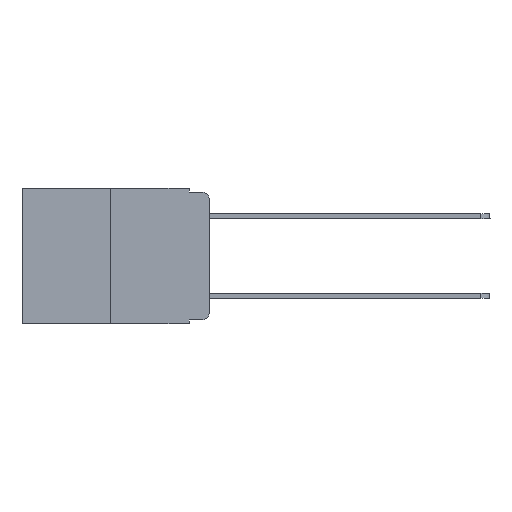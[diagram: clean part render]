
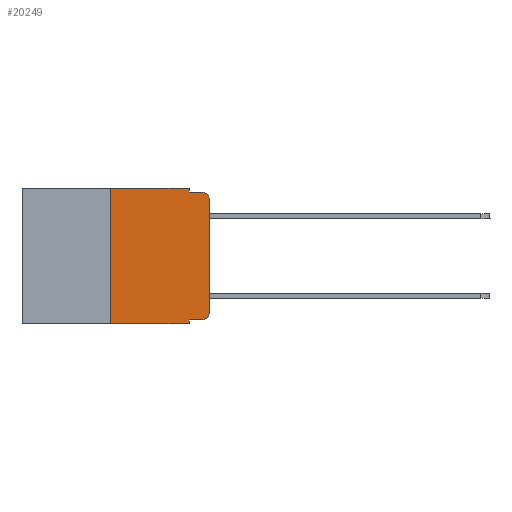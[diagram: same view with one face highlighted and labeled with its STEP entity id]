
A CAD part, left-side view. The second image highlights one B-rep face of the part: STEP entity #20249.
In plain terms, the highlighted planar face has unit normal (-1, 0, 0).
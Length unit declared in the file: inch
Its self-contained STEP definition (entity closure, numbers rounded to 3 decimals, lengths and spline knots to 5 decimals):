
#166 = ORIENTED_EDGE ( 'NONE', *, *, #11618, .F. ) ;
#709 = DIRECTION ( 'NONE',  ( 0., 0., -1. ) ) ;
#1634 = LINE ( 'NONE', #14642, #17639 ) ;
#1805 = DIRECTION ( 'NONE',  ( 0., 0., -1. ) ) ;
#2000 = CARTESIAN_POINT ( 'NONE',  ( 0., 0.473, 0. ) ) ;
#2023 = CARTESIAN_POINT ( 'NONE',  ( 0., 0.25, -0.343 ) ) ;
#2634 = DIRECTION ( 'NONE',  ( 0., -1., 0. ) ) ;
#2827 = CARTESIAN_POINT ( 'NONE',  ( 0., 0.25, 0. ) ) ;
#2883 = CARTESIAN_POINT ( 'NONE',  ( 0., 0.051, -0.343 ) ) ;
#2900 = CARTESIAN_POINT ( 'NONE',  ( 0., 0.051, -0.333 ) ) ;
#2901 = CARTESIAN_POINT ( 'NONE',  ( 0., 0.02, -0.333 ) ) ;
#3728 = CARTESIAN_POINT ( 'NONE',  ( 0., 0., -0.313 ) ) ;
#3731 = CIRCLE ( 'NONE', #4537, 0.02 ) ;
#3803 = ORIENTED_EDGE ( 'NONE', *, *, #8264, .F. ) ;
#3992 = VERTEX_POINT ( 'NONE', #2901 ) ;
#4128 = DIRECTION ( 'NONE',  ( -1., 0., 0. ) ) ;
#4416 = CARTESIAN_POINT ( 'NONE',  ( 0., 0.02, -0.313 ) ) ;
#4537 = AXIS2_PLACEMENT_3D ( 'NONE', #4416, #4580, #709 ) ;
#4580 = DIRECTION ( 'NONE',  ( -1., 0., 0. ) ) ;
#5114 = ORIENTED_EDGE ( 'NONE', *, *, #7189, .F. ) ;
#5396 = CARTESIAN_POINT ( 'NONE',  ( 0., 0.051, 0. ) ) ;
#5614 = EDGE_CURVE ( 'NONE', #18239, #15077, #23805, .T. ) ;
#6488 = DIRECTION ( 'NONE',  ( 0., -1., 0. ) ) ;
#6536 = ORIENTED_EDGE ( 'NONE', *, *, #17992, .F. ) ;
#6770 = DIRECTION ( 'NONE',  ( 0., 0., -1. ) ) ;
#6808 = ORIENTED_EDGE ( 'NONE', *, *, #16157, .F. ) ;
#7189 = EDGE_CURVE ( 'NONE', #14477, #15077, #16573, .T. ) ;
#8081 = CARTESIAN_POINT ( 'NONE',  ( 0., 0.25, 0. ) ) ;
#8264 = EDGE_CURVE ( 'NONE', #18609, #8531, #9358, .T. ) ;
#8531 = VERTEX_POINT ( 'NONE', #2883 ) ;
#8640 = VERTEX_POINT ( 'NONE', #3728 ) ;
#8918 = LINE ( 'NONE', #8081, #15441 ) ;
#8954 = DIRECTION ( 'NONE',  ( 0., 0., 1. ) ) ;
#9109 = CARTESIAN_POINT ( 'NONE',  ( 0., 0., 0. ) ) ;
#9358 = LINE ( 'NONE', #5396, #10633 ) ;
#10253 = DIRECTION ( 'NONE',  ( 0., 0., 1. ) ) ;
#10358 = CARTESIAN_POINT ( 'NONE',  ( 0., 0.051, -0.333 ) ) ;
#10443 = LINE ( 'NONE', #9109, #14481 ) ;
#10575 = VERTEX_POINT ( 'NONE', #2827 ) ;
#10633 = VECTOR ( 'NONE', #15311, 39.37008 ) ;
#10645 = DIRECTION ( 'NONE',  ( 0., -1., 0. ) ) ;
#11048 = CARTESIAN_POINT ( 'NONE',  ( 0., 0.02, -0.01 ) ) ;
#11168 = ORIENTED_EDGE ( 'NONE', *, *, #16854, .T. ) ;
#11304 = VECTOR ( 'NONE', #15984, 39.37008 ) ;
#11618 = EDGE_CURVE ( 'NONE', #10575, #21230, #24964, .T. ) ;
#11977 = PLANE ( 'NONE',  #17399 ) ;
#12824 = EDGE_CURVE ( 'NONE', #15800, #8531, #15035, .T. ) ;
#13599 = FACE_OUTER_BOUND ( 'NONE', #18260, .T. ) ;
#14142 = DIRECTION ( 'NONE',  ( 1., 0., 0. ) ) ;
#14287 = EDGE_CURVE ( 'NONE', #18609, #3992, #20779, .T. ) ;
#14477 = VERTEX_POINT ( 'NONE', #16768 ) ;
#14481 = VECTOR ( 'NONE', #8954, 39.37008 ) ;
#14642 = CARTESIAN_POINT ( 'NONE',  ( 0., 0.051, 0. ) ) ;
#14908 = CARTESIAN_POINT ( 'NONE',  ( 0., 0.051, 0. ) ) ;
#15035 = LINE ( 'NONE', #24073, #11304 ) ;
#15077 = VERTEX_POINT ( 'NONE', #11048 ) ;
#15311 = DIRECTION ( 'NONE',  ( 0., 0., -1. ) ) ;
#15441 = VECTOR ( 'NONE', #10253, 39.37008 ) ;
#15800 = VERTEX_POINT ( 'NONE', #2023 ) ;
#15944 = ORIENTED_EDGE ( 'NONE', *, *, #14287, .T. ) ;
#15984 = DIRECTION ( 'NONE',  ( 0., -1., 0. ) ) ;
#16157 = EDGE_CURVE ( 'NONE', #15800, #10575, #8918, .T. ) ;
#16573 = LINE ( 'NONE', #22268, #21773 ) ;
#16768 = CARTESIAN_POINT ( 'NONE',  ( 0., 0.051, -0.01 ) ) ;
#16854 = EDGE_CURVE ( 'NONE', #8640, #18239, #10443, .T. ) ;
#17399 = AXIS2_PLACEMENT_3D ( 'NONE', #2000, #14142, #21624 ) ;
#17639 = VECTOR ( 'NONE', #6770, 39.37008 ) ;
#17992 = EDGE_CURVE ( 'NONE', #21230, #14477, #1634, .T. ) ;
#18239 = VERTEX_POINT ( 'NONE', #23474 ) ;
#18260 = EDGE_LOOP ( 'NONE', ( #11168, #21896, #5114, #6536, #166, #6808, #18388, #3803, #15944, #19343 ) ) ;
#18388 = ORIENTED_EDGE ( 'NONE', *, *, #12824, .T. ) ;
#18478 = AXIS2_PLACEMENT_3D ( 'NONE', #21762, #4128, #1805 ) ;
#18609 = VERTEX_POINT ( 'NONE', #10358 ) ;
#19094 = VECTOR ( 'NONE', #10645, 39.37008 ) ;
#19220 = VECTOR ( 'NONE', #6488, 39.37008 ) ;
#19343 = ORIENTED_EDGE ( 'NONE', *, *, #20328, .T. ) ;
#20249 = ADVANCED_FACE ( 'NONE', ( #13599 ), #11977, .F. ) ;
#20328 = EDGE_CURVE ( 'NONE', #3992, #8640, #3731, .T. ) ;
#20779 = LINE ( 'NONE', #2900, #19220 ) ;
#21230 = VERTEX_POINT ( 'NONE', #14908 ) ;
#21624 = DIRECTION ( 'NONE',  ( 0., 0., -1. ) ) ;
#21762 = CARTESIAN_POINT ( 'NONE',  ( 0., 0.02, -0.03 ) ) ;
#21773 = VECTOR ( 'NONE', #2634, 39.37008 ) ;
#21835 = CARTESIAN_POINT ( 'NONE',  ( 0., 0.473, 0. ) ) ;
#21896 = ORIENTED_EDGE ( 'NONE', *, *, #5614, .T. ) ;
#22268 = CARTESIAN_POINT ( 'NONE',  ( 0., 0.051, -0.01 ) ) ;
#23474 = CARTESIAN_POINT ( 'NONE',  ( 0., 0., -0.03 ) ) ;
#23805 = CIRCLE ( 'NONE', #18478, 0.02 ) ;
#24073 = CARTESIAN_POINT ( 'NONE',  ( 0., 0.473, -0.343 ) ) ;
#24964 = LINE ( 'NONE', #21835, #19094 ) ;
